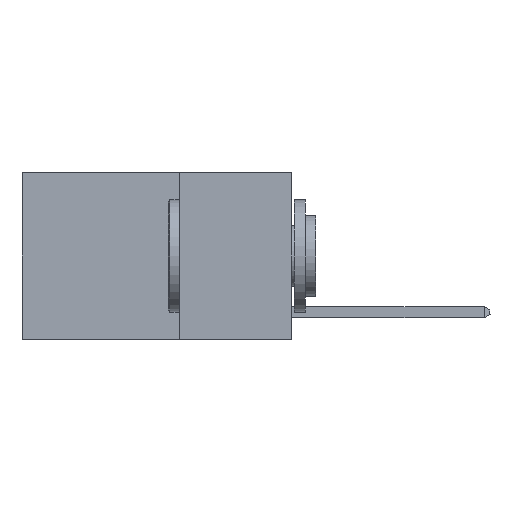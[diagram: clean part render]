
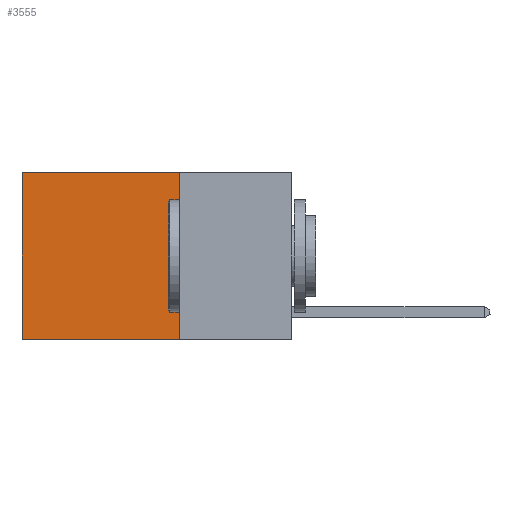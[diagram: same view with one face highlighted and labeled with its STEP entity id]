
A CAD part, left-side view. The second image highlights one B-rep face of the part: STEP entity #3555.
In plain terms, the highlighted planar face has unit normal (-1, 0, 0).
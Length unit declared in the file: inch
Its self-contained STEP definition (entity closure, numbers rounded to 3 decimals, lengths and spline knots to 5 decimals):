
#1003 = EDGE_CURVE ( 'NONE', #4553, #19789, #20850, .T. ) ;
#1088 = VECTOR ( 'NONE', #5795, 39.37008 ) ;
#1275 = ORIENTED_EDGE ( 'NONE', *, *, #1003, .F. ) ;
#3172 = CARTESIAN_POINT ( 'NONE',  ( 0.2625, 0.25, -0.37 ) ) ;
#3555 = ADVANCED_FACE ( 'NONE', ( #7248 ), #7024, .F. ) ;
#4553 = VERTEX_POINT ( 'NONE', #8021 ) ;
#4578 = LINE ( 'NONE', #15298, #8684 ) ;
#5067 = CARTESIAN_POINT ( 'NONE',  ( 0.2625, 0.25, 0. ) ) ;
#5795 = DIRECTION ( 'NONE',  ( 0., 1., 0. ) ) ;
#5917 = AXIS2_PLACEMENT_3D ( 'NONE', #14044, #10354, #8631 ) ;
#6704 = EDGE_CURVE ( 'NONE', #4553, #18800, #9104, .T. ) ;
#6885 = LINE ( 'NONE', #17046, #16665 ) ;
#6908 = DIRECTION ( 'NONE',  ( 0., 0., -1. ) ) ;
#7024 = PLANE ( 'NONE',  #5917 ) ;
#7129 = ORIENTED_EDGE ( 'NONE', *, *, #22326, .F. ) ;
#7248 = FACE_OUTER_BOUND ( 'NONE', #14164, .T. ) ;
#7346 = VECTOR ( 'NONE', #6908, 39.37008 ) ;
#8021 = CARTESIAN_POINT ( 'NONE',  ( 0.2625, 0.25, 0. ) ) ;
#8631 = DIRECTION ( 'NONE',  ( 0., 0., -1. ) ) ;
#8684 = VECTOR ( 'NONE', #22670, 39.37008 ) ;
#9104 = LINE ( 'NONE', #12684, #1088 ) ;
#10295 = CARTESIAN_POINT ( 'NONE',  ( 0.2625, 0.6, 0. ) ) ;
#10354 = DIRECTION ( 'NONE',  ( 1., 0., 0. ) ) ;
#11294 = EDGE_CURVE ( 'NONE', #18800, #19534, #6885, .T. ) ;
#12684 = CARTESIAN_POINT ( 'NONE',  ( 0.2625, 0.25, 0. ) ) ;
#13961 = ORIENTED_EDGE ( 'NONE', *, *, #11294, .T. ) ;
#14044 = CARTESIAN_POINT ( 'NONE',  ( 0.2625, 0.25, 0. ) ) ;
#14164 = EDGE_LOOP ( 'NONE', ( #13961, #7129, #1275, #16933 ) ) ;
#15298 = CARTESIAN_POINT ( 'NONE',  ( 0.2625, 0.25, -0.37 ) ) ;
#15556 = DIRECTION ( 'NONE',  ( 0., 0., -1. ) ) ;
#16665 = VECTOR ( 'NONE', #15556, 39.37008 ) ;
#16933 = ORIENTED_EDGE ( 'NONE', *, *, #6704, .T. ) ;
#17046 = CARTESIAN_POINT ( 'NONE',  ( 0.2625, 0.6, 0. ) ) ;
#18317 = CARTESIAN_POINT ( 'NONE',  ( 0.2625, 0.6, -0.37 ) ) ;
#18800 = VERTEX_POINT ( 'NONE', #10295 ) ;
#19534 = VERTEX_POINT ( 'NONE', #18317 ) ;
#19789 = VERTEX_POINT ( 'NONE', #3172 ) ;
#20850 = LINE ( 'NONE', #5067, #7346 ) ;
#22326 = EDGE_CURVE ( 'NONE', #19789, #19534, #4578, .T. ) ;
#22670 = DIRECTION ( 'NONE',  ( 0., 1., 0. ) ) ;
